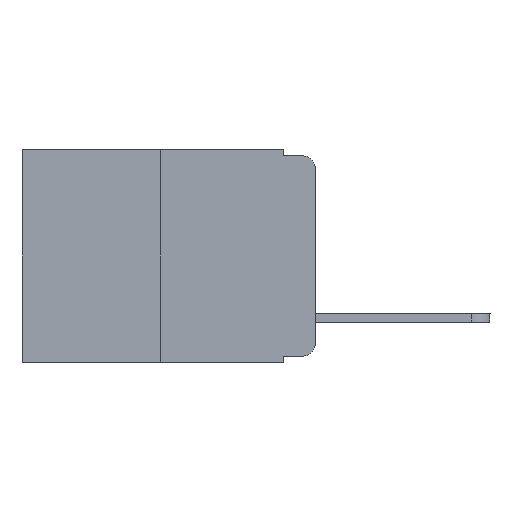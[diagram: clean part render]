
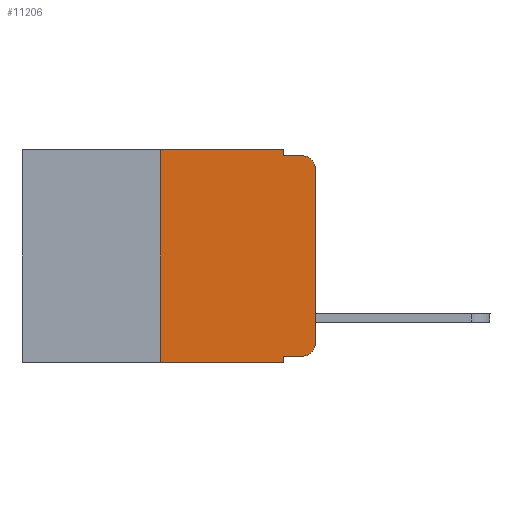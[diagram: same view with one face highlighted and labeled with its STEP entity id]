
A CAD part, left-side view. The second image highlights one B-rep face of the part: STEP entity #11206.
In plain terms, the highlighted planar face has unit normal (-1, 0, 0).
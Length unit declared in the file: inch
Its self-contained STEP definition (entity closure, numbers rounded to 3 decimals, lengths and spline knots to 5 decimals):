
#203 = EDGE_CURVE ( 'NONE', #12398, #251, #4345, .T. ) ;
#251 = VERTEX_POINT ( 'NONE', #15795 ) ;
#427 = CARTESIAN_POINT ( 'NONE',  ( 0., 0., 0. ) ) ;
#629 = CARTESIAN_POINT ( 'NONE',  ( 0., 0.051, -0.01 ) ) ;
#643 = CARTESIAN_POINT ( 'NONE',  ( 0., 0.473, 0. ) ) ;
#840 = VERTEX_POINT ( 'NONE', #10516 ) ;
#989 = LINE ( 'NONE', #643, #11000 ) ;
#1278 = EDGE_CURVE ( 'NONE', #840, #4118, #2856, .T. ) ;
#1980 = DIRECTION ( 'NONE',  ( -1., 0., 0. ) ) ;
#2025 = CARTESIAN_POINT ( 'NONE',  ( 0., 0.051, 0. ) ) ;
#2224 = ORIENTED_EDGE ( 'NONE', *, *, #17625, .F. ) ;
#2554 = VERTEX_POINT ( 'NONE', #19440 ) ;
#2692 = ORIENTED_EDGE ( 'NONE', *, *, #203, .T. ) ;
#2856 = CIRCLE ( 'NONE', #6053, 0.02 ) ;
#2904 = CARTESIAN_POINT ( 'NONE',  ( 0., 0.25, 0. ) ) ;
#2978 = VECTOR ( 'NONE', #8331, 39.37008 ) ;
#3458 = DIRECTION ( 'NONE',  ( 0., 0., -1. ) ) ;
#3528 = DIRECTION ( 'NONE',  ( -1., 0., 0. ) ) ;
#4118 = VERTEX_POINT ( 'NONE', #17647 ) ;
#4345 = CIRCLE ( 'NONE', #17621, 0.02 ) ;
#4767 = EDGE_LOOP ( 'NONE', ( #19805, #5729, #10357, #14203, #2224, #13946, #15404, #19707, #17001, #2692 ) ) ;
#4886 = CARTESIAN_POINT ( 'NONE',  ( 0., 0.02, -0.03 ) ) ;
#5156 = DIRECTION ( 'NONE',  ( 0., -1., 0. ) ) ;
#5276 = DIRECTION ( 'NONE',  ( 0., 0., 1. ) ) ;
#5414 = EDGE_CURVE ( 'NONE', #10853, #12398, #18139, .T. ) ;
#5729 = ORIENTED_EDGE ( 'NONE', *, *, #1278, .T. ) ;
#5730 = CARTESIAN_POINT ( 'NONE',  ( 0., 0.051, 0. ) ) ;
#6053 = AXIS2_PLACEMENT_3D ( 'NONE', #4886, #3528, #3458 ) ;
#6508 = VECTOR ( 'NONE', #5276, 39.37008 ) ;
#6584 = CARTESIAN_POINT ( 'NONE',  ( 0., 0.473, 0. ) ) ;
#6707 = DIRECTION ( 'NONE',  ( 0., -1., 0. ) ) ;
#7392 = VECTOR ( 'NONE', #19559, 39.37008 ) ;
#7599 = EDGE_CURVE ( 'NONE', #9972, #15451, #10583, .T. ) ;
#8331 = DIRECTION ( 'NONE',  ( 0., -1., 0. ) ) ;
#8629 = VECTOR ( 'NONE', #11410, 39.37008 ) ;
#9102 = LINE ( 'NONE', #427, #8629 ) ;
#9519 = EDGE_CURVE ( 'NONE', #10853, #2554, #19420, .T. ) ;
#9771 = CARTESIAN_POINT ( 'NONE',  ( 0., 0.02, -0.333 ) ) ;
#9972 = VERTEX_POINT ( 'NONE', #11882 ) ;
#10357 = ORIENTED_EDGE ( 'NONE', *, *, #18236, .F. ) ;
#10516 = CARTESIAN_POINT ( 'NONE',  ( 0., 0., -0.03 ) ) ;
#10583 = LINE ( 'NONE', #11269, #6508 ) ;
#10700 = VERTEX_POINT ( 'NONE', #15809 ) ;
#10853 = VERTEX_POINT ( 'NONE', #11866 ) ;
#11000 = VECTOR ( 'NONE', #6707, 39.37008 ) ;
#11181 = PLANE ( 'NONE',  #19560 ) ;
#11206 = ADVANCED_FACE ( 'NONE', ( #13937 ), #11181, .F. ) ;
#11247 = DIRECTION ( 'NONE',  ( 0., 0., -1. ) ) ;
#11269 = CARTESIAN_POINT ( 'NONE',  ( 0., 0.25, 0. ) ) ;
#11410 = DIRECTION ( 'NONE',  ( 0., 0., 1. ) ) ;
#11693 = LINE ( 'NONE', #629, #14366 ) ;
#11866 = CARTESIAN_POINT ( 'NONE',  ( 0., 0.051, -0.333 ) ) ;
#11882 = CARTESIAN_POINT ( 'NONE',  ( 0., 0.25, -0.343 ) ) ;
#12398 = VERTEX_POINT ( 'NONE', #9771 ) ;
#12436 = EDGE_CURVE ( 'NONE', #251, #840, #9102, .T. ) ;
#12537 = CARTESIAN_POINT ( 'NONE',  ( 0., 0.02, -0.313 ) ) ;
#12741 = DIRECTION ( 'NONE',  ( 0., 0., -1. ) ) ;
#12754 = DIRECTION ( 'NONE',  ( 0., 0., -1. ) ) ;
#13195 = DIRECTION ( 'NONE',  ( 0., -1., 0. ) ) ;
#13762 = VERTEX_POINT ( 'NONE', #13950 ) ;
#13937 = FACE_OUTER_BOUND ( 'NONE', #4767, .T. ) ;
#13946 = ORIENTED_EDGE ( 'NONE', *, *, #7599, .F. ) ;
#13950 = CARTESIAN_POINT ( 'NONE',  ( 0., 0.051, -0.01 ) ) ;
#14203 = ORIENTED_EDGE ( 'NONE', *, *, #19044, .F. ) ;
#14366 = VECTOR ( 'NONE', #5156, 39.37008 ) ;
#14544 = VECTOR ( 'NONE', #13195, 39.37008 ) ;
#15320 = VECTOR ( 'NONE', #11247, 39.37008 ) ;
#15404 = ORIENTED_EDGE ( 'NONE', *, *, #19542, .T. ) ;
#15451 = VERTEX_POINT ( 'NONE', #2904 ) ;
#15795 = CARTESIAN_POINT ( 'NONE',  ( 0., 0., -0.313 ) ) ;
#15809 = CARTESIAN_POINT ( 'NONE',  ( 0., 0.051, 0. ) ) ;
#16368 = CARTESIAN_POINT ( 'NONE',  ( 0., 0.473, -0.343 ) ) ;
#17001 = ORIENTED_EDGE ( 'NONE', *, *, #5414, .T. ) ;
#17621 = AXIS2_PLACEMENT_3D ( 'NONE', #12537, #1980, #12754 ) ;
#17625 = EDGE_CURVE ( 'NONE', #15451, #10700, #989, .T. ) ;
#17647 = CARTESIAN_POINT ( 'NONE',  ( 0., 0.02, -0.01 ) ) ;
#17715 = LINE ( 'NONE', #5730, #7392 ) ;
#18139 = LINE ( 'NONE', #18935, #2978 ) ;
#18177 = LINE ( 'NONE', #16368, #14544 ) ;
#18236 = EDGE_CURVE ( 'NONE', #13762, #4118, #11693, .T. ) ;
#18816 = DIRECTION ( 'NONE',  ( 1., 0., 0. ) ) ;
#18935 = CARTESIAN_POINT ( 'NONE',  ( 0., 0.051, -0.333 ) ) ;
#19044 = EDGE_CURVE ( 'NONE', #10700, #13762, #17715, .T. ) ;
#19420 = LINE ( 'NONE', #2025, #15320 ) ;
#19440 = CARTESIAN_POINT ( 'NONE',  ( 0., 0.051, -0.343 ) ) ;
#19542 = EDGE_CURVE ( 'NONE', #9972, #2554, #18177, .T. ) ;
#19559 = DIRECTION ( 'NONE',  ( 0., 0., -1. ) ) ;
#19560 = AXIS2_PLACEMENT_3D ( 'NONE', #6584, #18816, #12741 ) ;
#19707 = ORIENTED_EDGE ( 'NONE', *, *, #9519, .F. ) ;
#19805 = ORIENTED_EDGE ( 'NONE', *, *, #12436, .T. ) ;
